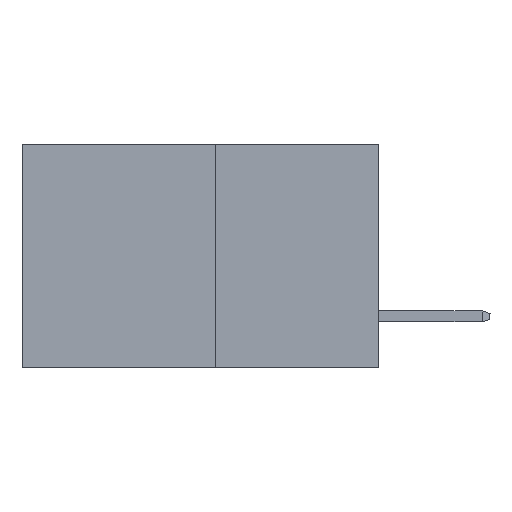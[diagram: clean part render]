
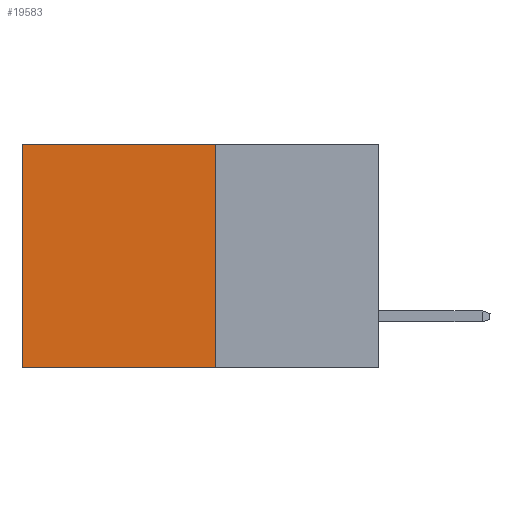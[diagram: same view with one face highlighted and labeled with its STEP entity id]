
A CAD part, left-side view. The second image highlights one B-rep face of the part: STEP entity #19583.
In plain terms, the highlighted planar face has unit normal (-1, 0, 0).
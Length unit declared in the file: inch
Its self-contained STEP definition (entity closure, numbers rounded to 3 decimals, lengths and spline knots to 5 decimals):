
#355 = EDGE_CURVE ( 'NONE', #10981, #4348, #15515, .T. ) ;
#1029 = CARTESIAN_POINT ( 'NONE',  ( 0.277, 0.27, -0.37 ) ) ;
#1554 = AXIS2_PLACEMENT_3D ( 'NONE', #23217, #9898, #25383 ) ;
#2096 = FACE_OUTER_BOUND ( 'NONE', #22187, .T. ) ;
#3356 = ORIENTED_EDGE ( 'NONE', *, *, #9970, .F. ) ;
#3499 = VECTOR ( 'NONE', #11278, 39.37008 ) ;
#4348 = VERTEX_POINT ( 'NONE', #28392 ) ;
#5179 = ORIENTED_EDGE ( 'NONE', *, *, #22202, .T. ) ;
#5401 = DIRECTION ( 'NONE',  ( 0., 1., 0. ) ) ;
#9898 = DIRECTION ( 'NONE',  ( 1., 0., 0. ) ) ;
#9970 = EDGE_CURVE ( 'NONE', #13370, #24305, #18802, .T. ) ;
#10774 = LINE ( 'NONE', #25014, #21899 ) ;
#10981 = VERTEX_POINT ( 'NONE', #26491 ) ;
#11278 = DIRECTION ( 'NONE',  ( 0., 1., 0. ) ) ;
#11334 = DIRECTION ( 'NONE',  ( 0., 0., -1. ) ) ;
#11680 = ORIENTED_EDGE ( 'NONE', *, *, #25970, .F. ) ;
#13370 = VERTEX_POINT ( 'NONE', #22602 ) ;
#15373 = LINE ( 'NONE', #24570, #20542 ) ;
#15515 = LINE ( 'NONE', #24271, #3499 ) ;
#18802 = LINE ( 'NONE', #1029, #23932 ) ;
#18809 = PLANE ( 'NONE',  #1554 ) ;
#19004 = ORIENTED_EDGE ( 'NONE', *, *, #355, .T. ) ;
#19127 = CARTESIAN_POINT ( 'NONE',  ( 0.277, 0.59, -0.37 ) ) ;
#19583 = ADVANCED_FACE ( 'NONE', ( #2096 ), #18809, .F. ) ;
#20542 = VECTOR ( 'NONE', #11334, 39.37008 ) ;
#21899 = VECTOR ( 'NONE', #27162, 39.37008 ) ;
#22187 = EDGE_LOOP ( 'NONE', ( #5179, #3356, #11680, #19004 ) ) ;
#22202 = EDGE_CURVE ( 'NONE', #4348, #24305, #10774, .T. ) ;
#22602 = CARTESIAN_POINT ( 'NONE',  ( 0.277, 0.27, -0.37 ) ) ;
#23217 = CARTESIAN_POINT ( 'NONE',  ( 0.277, 0.27, -0.37 ) ) ;
#23932 = VECTOR ( 'NONE', #5401, 39.37008 ) ;
#24271 = CARTESIAN_POINT ( 'NONE',  ( 0.277, 0.27, 0. ) ) ;
#24305 = VERTEX_POINT ( 'NONE', #19127 ) ;
#24570 = CARTESIAN_POINT ( 'NONE',  ( 0.277, 0.27, -0.37 ) ) ;
#25014 = CARTESIAN_POINT ( 'NONE',  ( 0.277, 0.59, -0.37 ) ) ;
#25383 = DIRECTION ( 'NONE',  ( 0., 0., -1. ) ) ;
#25970 = EDGE_CURVE ( 'NONE', #10981, #13370, #15373, .T. ) ;
#26491 = CARTESIAN_POINT ( 'NONE',  ( 0.277, 0.27, 0. ) ) ;
#27162 = DIRECTION ( 'NONE',  ( 0., 0., -1. ) ) ;
#28392 = CARTESIAN_POINT ( 'NONE',  ( 0.277, 0.59, 0. ) ) ;
